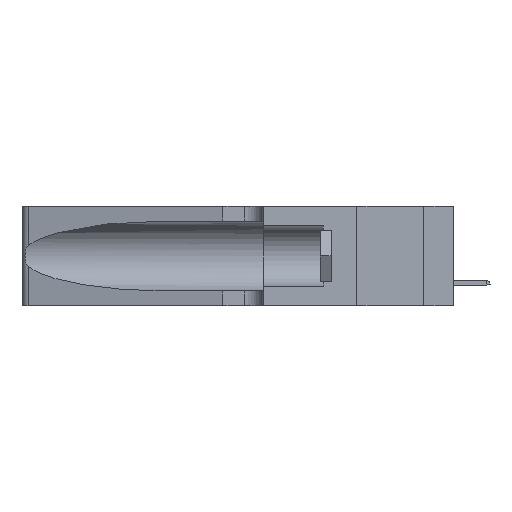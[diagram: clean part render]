
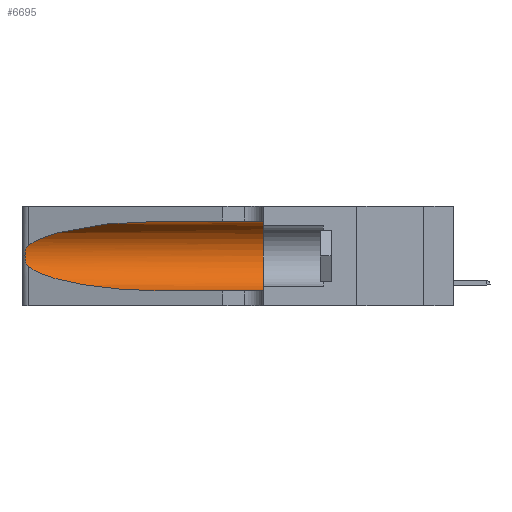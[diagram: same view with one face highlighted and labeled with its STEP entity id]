
A CAD part, left-side view. The second image highlights one B-rep face of the part: STEP entity #6695.
In plain terms, the highlighted cylindrical face has radius 3.308 mm (diameter 6.617 mm), a partial arc.
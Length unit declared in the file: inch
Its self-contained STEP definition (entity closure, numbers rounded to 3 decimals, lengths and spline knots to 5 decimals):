
#199 = CARTESIAN_POINT ( 'NONE',  ( 0.25555, 1.22994, 0.2215 ) ) ;
#1051 = VERTEX_POINT ( 'NONE', #31747 ) ;
#1526 = DIRECTION ( 'NONE',  ( 0., -1., 0. ) ) ;
#2728 = DIRECTION ( 'NONE',  ( 0., 0., -1. ) ) ;
#2874 = CARTESIAN_POINT ( 'NONE',  ( 0.1305, 0.35, 0.05475 ) ) ;
#2947 = VERTEX_POINT ( 'NONE', #29113 ) ;
#3472 = CARTESIAN_POINT ( 'NONE',  ( 0.18966, 0.96281, 0.05475 ) ) ;
#4172 = VERTEX_POINT ( 'NONE', #2874 ) ;
#4754 = CARTESIAN_POINT ( 'NONE',  ( 0.1305, 1.61858, 0.31525 ) ) ;
#4791 = CARTESIAN_POINT ( 'NONE',  ( 0.2373, 1.15595, 0.28018 ) ) ;
#5012 = CARTESIAN_POINT ( 'NONE',  ( 0.25487, 1.22718, 0.22369 ) ) ;
#6235 = DIRECTION ( 'NONE',  ( 0., 0., 1. ) ) ;
#6374 = DIRECTION ( 'NONE',  ( 0., -1., 0. ) ) ;
#6695 = ADVANCED_FACE ( 'NONE', ( #19145 ), #32266, .F. ) ;
#6872 = CARTESIAN_POINT ( 'NONE',  ( 0.26075, 1.23896, 0.178 ) ) ;
#7155 = AXIS2_PLACEMENT_3D ( 'NONE', #15328, #29120, #6235 ) ;
#7305 = CARTESIAN_POINT ( 'NONE',  ( 0.25854, 1.2359, 0.20912 ) ) ;
#7514 = CARTESIAN_POINT ( 'NONE',  ( 0.25789, 1.23486, 0.15765 ) ) ;
#7829 = VERTEX_POINT ( 'NONE', #32291 ) ;
#10414 = VERTEX_POINT ( 'NONE', #23453 ) ;
#10774 = CARTESIAN_POINT ( 'NONE',  ( 0.25787, 1.23484, 0.2124 ) ) ;
#10977 = CARTESIAN_POINT ( 'NONE',  ( 0.25856, 1.23593, 0.16098 ) ) ;
#12982 = CARTESIAN_POINT ( 'NONE',  ( 0.1305, 0.72297, 0.05475 ) ) ;
#14226 = CARTESIAN_POINT ( 'NONE',  ( 0.25487, 1.22718, 0.22369 ) ) ;
#14337 = VECTOR ( 'NONE', #37445, 39.37008 ) ;
#14638 = VECTOR ( 'NONE', #1526, 39.37008 ) ;
#15328 = CARTESIAN_POINT ( 'NONE',  ( 0.1305, 0.35, 0.185 ) ) ;
#15370 = CARTESIAN_POINT ( 'NONE',  ( 0.18966, 0.96281, 0.31525 ) ) ;
#17130 = ORIENTED_EDGE ( 'NONE', *, *, #22636, .F. ) ;
#17738 = AXIS2_PLACEMENT_3D ( 'NONE', #38336, #6374, #2728 ) ;
#18489 = ORIENTED_EDGE ( 'NONE', *, *, #26835, .T. ) ;
#18709 = EDGE_CURVE ( 'NONE', #2947, #7829, #24825, .T. ) ;
#19145 = FACE_OUTER_BOUND ( 'NONE', #40512, .T. ) ;
#20060 = CARTESIAN_POINT ( 'NONE',  ( 0.25639, 1.23186, 0.15144 ) ) ;
#20104 = CARTESIAN_POINT ( 'NONE',  ( 0.25487, 1.22718, 0.14631 ) ) ;
#20707 = CARTESIAN_POINT ( 'NONE',  ( 0.25555, 1.22993, 0.14849 ) ) ;
#22636 = EDGE_CURVE ( 'NONE', #7829, #4172, #27885, .T. ) ;
#23295 = CARTESIAN_POINT ( 'NONE',  ( 0.25639, 1.23184, 0.21858 ) ) ;
#23453 = CARTESIAN_POINT ( 'NONE',  ( 0.1305, 0.72297, 0.05475 ) ) ;
#23931 = CARTESIAN_POINT ( 'NONE',  ( 0.26017, 1.23833, 0.17102 ) ) ;
#24825 = LINE ( 'NONE', #4754, #14638 ) ;
#26835 = EDGE_CURVE ( 'NONE', #37443, #10414, #38008, .T. ) ;
#26953 = CARTESIAN_POINT ( 'NONE',  ( 0.25487, 1.22718, 0.14631 ) ) ;
#27885 = CIRCLE ( 'NONE', #7155, 0.13025 ) ;
#29113 = CARTESIAN_POINT ( 'NONE',  ( 0.1305, 0.72297, 0.31525 ) ) ;
#29120 = DIRECTION ( 'NONE',  ( 0., 1., 0. ) ) ;
#29191 =( BOUNDED_CURVE ( )  B_SPLINE_CURVE ( 3, ( #34553, #15370, #4791, #5012 ),
 .UNSPECIFIED., .F., .F. ) 
 B_SPLINE_CURVE_WITH_KNOTS ( ( 4, 4 ),
 ( 1.5708, 2.84003 ),
 .UNSPECIFIED. ) 
 CURVE ( )  GEOMETRIC_REPRESENTATION_ITEM ( )  RATIONAL_B_SPLINE_CURVE ( ( 1., 0.87, 0.87, 1. ) ) 
 REPRESENTATION_ITEM ( '' )  );
#29597 = ORIENTED_EDGE ( 'NONE', *, *, #39744, .T. ) ;
#30685 = EDGE_CURVE ( 'NONE', #2947, #1051, #29191, .T. ) ;
#31747 = CARTESIAN_POINT ( 'NONE',  ( 0.25487, 1.22718, 0.22369 ) ) ;
#32266 = CYLINDRICAL_SURFACE ( 'NONE', #17738, 0.13025 ) ;
#32291 = CARTESIAN_POINT ( 'NONE',  ( 0.1305, 0.35, 0.31525 ) ) ;
#32319 = ORIENTED_EDGE ( 'NONE', *, *, #30685, .T. ) ;
#34553 = CARTESIAN_POINT ( 'NONE',  ( 0.1305, 0.72297, 0.31525 ) ) ;
#35420 = B_SPLINE_CURVE_WITH_KNOTS ( 'NONE', 3,
 ( #14226, #199, #23295, #10774, #7305, #39675, #40537, #6872, #23931, #10977, #7514, #20060, #20707, #26953 ),
 .UNSPECIFIED., .F., .F.,
 ( 4, 2, 2, 2, 2, 2, 4 ),
 ( 0., 0.00027, 0.00053, 0.00107, 0.0016, 0.00187, 0.00214 ),
 .UNSPECIFIED. ) ;
#35573 = ORIENTED_EDGE ( 'NONE', *, *, #39085, .T. ) ;
#37178 = ORIENTED_EDGE ( 'NONE', *, *, #18709, .F. ) ;
#37443 = VERTEX_POINT ( 'NONE', #39559 ) ;
#37445 = DIRECTION ( 'NONE',  ( 0., -1., 0. ) ) ;
#37666 = CARTESIAN_POINT ( 'NONE',  ( 0.1305, 1.61858, 0.05475 ) ) ;
#38008 =( BOUNDED_CURVE ( )  B_SPLINE_CURVE ( 3, ( #20104, #39926, #3472, #12982 ),
 .UNSPECIFIED., .F., .F. ) 
 B_SPLINE_CURVE_WITH_KNOTS ( ( 4, 4 ),
 ( 3.44316, 4.71239 ),
 .UNSPECIFIED. ) 
 CURVE ( )  GEOMETRIC_REPRESENTATION_ITEM ( )  RATIONAL_B_SPLINE_CURVE ( ( 1., 0.87, 0.87, 1. ) ) 
 REPRESENTATION_ITEM ( '' )  );
#38336 = CARTESIAN_POINT ( 'NONE',  ( 0.1305, 1.61858, 0.185 ) ) ;
#39085 = EDGE_CURVE ( 'NONE', #10414, #4172, #40678, .T. ) ;
#39559 = CARTESIAN_POINT ( 'NONE',  ( 0.25487, 1.22718, 0.14631 ) ) ;
#39675 = CARTESIAN_POINT ( 'NONE',  ( 0.26018, 1.23835, 0.19895 ) ) ;
#39744 = EDGE_CURVE ( 'NONE', #1051, #37443, #35420, .T. ) ;
#39926 = CARTESIAN_POINT ( 'NONE',  ( 0.2373, 1.15595, 0.08982 ) ) ;
#40512 = EDGE_LOOP ( 'NONE', ( #32319, #29597, #18489, #35573, #17130, #37178 ) ) ;
#40537 = CARTESIAN_POINT ( 'NONE',  ( 0.26075, 1.23896, 0.19203 ) ) ;
#40678 = LINE ( 'NONE', #37666, #14337 ) ;
